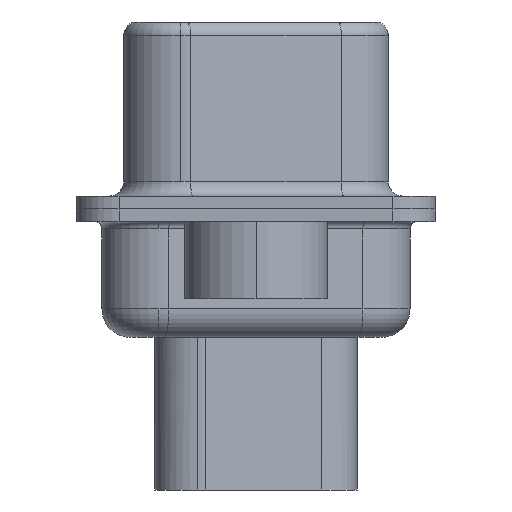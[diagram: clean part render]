
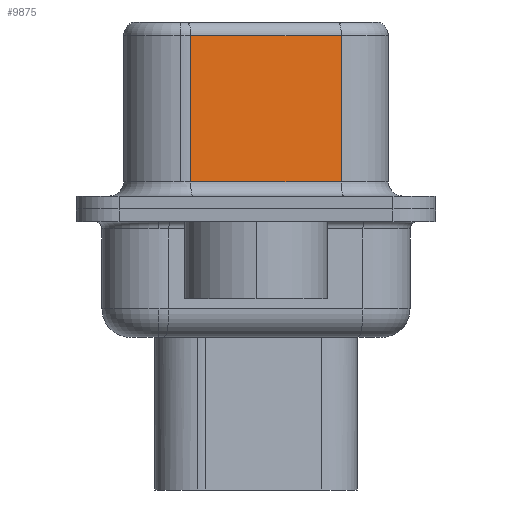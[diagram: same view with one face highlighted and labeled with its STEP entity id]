
A CAD part, left-side view. The second image highlights one B-rep face of the part: STEP entity #9875.
In plain terms, the highlighted planar face has unit normal (-0.985, -0.174, 0).
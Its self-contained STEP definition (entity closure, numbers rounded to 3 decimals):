
#777 = DIRECTION ( 'NONE',  ( 0.985, 0.174, 0. ) ) ;
#1554 = VERTEX_POINT ( 'NONE', #11433 ) ;
#2025 = EDGE_CURVE ( 'NONE', #13090, #22106, #20047, .T. ) ;
#2677 = LINE ( 'NONE', #9750, #14722 ) ;
#4343 = CARTESIAN_POINT ( 'NONE',  ( 4.551, -2.987, 6.57 ) ) ;
#5742 = VECTOR ( 'NONE', #20989, 1000. ) ;
#5848 = DIRECTION ( 'NONE',  ( -0.174, 0.985, 0. ) ) ;
#5860 = EDGE_CURVE ( 'NONE', #1554, #22106, #16673, .T. ) ;
#6655 = ORIENTED_EDGE ( 'NONE', *, *, #5860, .T. ) ;
#7208 = ORIENTED_EDGE ( 'NONE', *, *, #13261, .T. ) ;
#8440 = ORIENTED_EDGE ( 'NONE', *, *, #2025, .F. ) ;
#9750 = CARTESIAN_POINT ( 'NONE',  ( 4.551, -2.987, 6.07 ) ) ;
#9875 = ADVANCED_FACE ( 'NONE', ( #11065 ), #12924, .F. ) ;
#10476 = CARTESIAN_POINT ( 'NONE',  ( 3.62, 2.293, 6.07 ) ) ;
#11065 = FACE_OUTER_BOUND ( 'NONE', #15577, .T. ) ;
#11182 = DIRECTION ( 'NONE',  ( -0.174, 0.985, 0. ) ) ;
#11433 = CARTESIAN_POINT ( 'NONE',  ( 3.62, 2.293, 0.95 ) ) ;
#12601 = EDGE_CURVE ( 'NONE', #16608, #1554, #22199, .T. ) ;
#12924 = PLANE ( 'NONE',  #16149 ) ;
#13090 = VERTEX_POINT ( 'NONE', #13568 ) ;
#13261 = EDGE_CURVE ( 'NONE', #13090, #16608, #2677, .T. ) ;
#13568 = CARTESIAN_POINT ( 'NONE',  ( 4.551, -2.987, 6.07 ) ) ;
#13934 = DIRECTION ( 'NONE',  ( 0., 0., -1. ) ) ;
#13989 = CARTESIAN_POINT ( 'NONE',  ( 4.551, -2.987, 0.95 ) ) ;
#14722 = VECTOR ( 'NONE', #5848, 1000. ) ;
#15024 = ORIENTED_EDGE ( 'NONE', *, *, #12601, .T. ) ;
#15577 = EDGE_LOOP ( 'NONE', ( #8440, #7208, #15024, #6655 ) ) ;
#16149 = AXIS2_PLACEMENT_3D ( 'NONE', #18189, #777, #11182 ) ;
#16608 = VERTEX_POINT ( 'NONE', #10476 ) ;
#16660 = VECTOR ( 'NONE', #18328, 1000. ) ;
#16673 = LINE ( 'NONE', #13989, #5742 ) ;
#17250 = CARTESIAN_POINT ( 'NONE',  ( 3.62, 2.293, 6.57 ) ) ;
#17338 = VECTOR ( 'NONE', #13934, 1000. ) ;
#18189 = CARTESIAN_POINT ( 'NONE',  ( 4.551, -2.987, 6.57 ) ) ;
#18328 = DIRECTION ( 'NONE',  ( 0., 0., -1. ) ) ;
#20047 = LINE ( 'NONE', #4343, #16660 ) ;
#20360 = CARTESIAN_POINT ( 'NONE',  ( 4.551, -2.987, 0.95 ) ) ;
#20989 = DIRECTION ( 'NONE',  ( 0.174, -0.985, 0. ) ) ;
#22106 = VERTEX_POINT ( 'NONE', #20360 ) ;
#22199 = LINE ( 'NONE', #17250, #17338 ) ;
